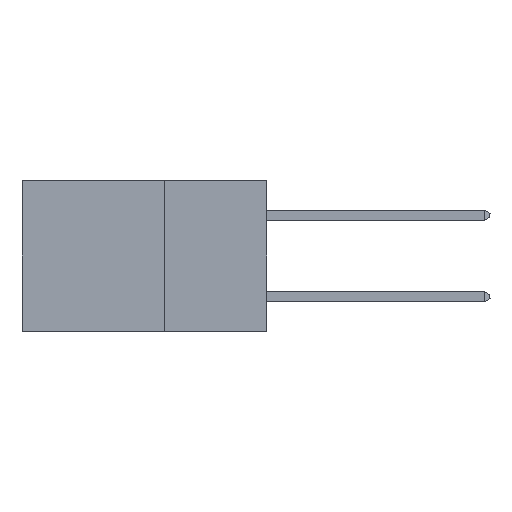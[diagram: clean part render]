
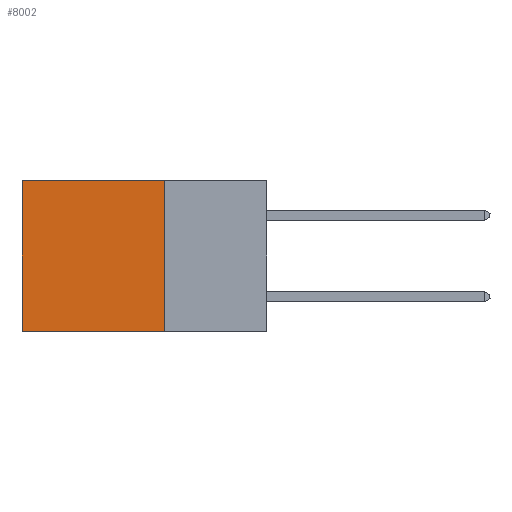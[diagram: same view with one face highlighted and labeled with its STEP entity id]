
A CAD part, left-side view. The second image highlights one B-rep face of the part: STEP entity #8002.
In plain terms, the highlighted planar face has unit normal (-1, 0, 0).
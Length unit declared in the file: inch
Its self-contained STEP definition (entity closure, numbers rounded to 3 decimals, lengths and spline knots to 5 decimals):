
#333 = DIRECTION ( 'NONE',  ( 0., 0., -1. ) ) ;
#363 = VERTEX_POINT ( 'NONE', #15415 ) ;
#1330 = ORIENTED_EDGE ( 'NONE', *, *, #5428, .T. ) ;
#1715 = DIRECTION ( 'NONE',  ( 0., 1., 0. ) ) ;
#1804 = VECTOR ( 'NONE', #1857, 39.37008 ) ;
#1857 = DIRECTION ( 'NONE',  ( 0., 0., -1. ) ) ;
#1871 = VERTEX_POINT ( 'NONE', #3184 ) ;
#2677 = LINE ( 'NONE', #12486, #1804 ) ;
#3184 = CARTESIAN_POINT ( 'NONE',  ( 0.2875, 0.25, 0. ) ) ;
#3220 = EDGE_CURVE ( 'NONE', #11445, #363, #10912, .T. ) ;
#3575 = VERTEX_POINT ( 'NONE', #6462 ) ;
#5428 = EDGE_CURVE ( 'NONE', #3575, #363, #2677, .T. ) ;
#6144 = AXIS2_PLACEMENT_3D ( 'NONE', #7206, #8565, #333 ) ;
#6462 = CARTESIAN_POINT ( 'NONE',  ( 0.2875, 0.6, 0. ) ) ;
#6562 = DIRECTION ( 'NONE',  ( 0., 1., 0. ) ) ;
#7206 = CARTESIAN_POINT ( 'NONE',  ( 0.2875, 0.25, 0. ) ) ;
#7434 = VECTOR ( 'NONE', #1715, 39.37008 ) ;
#8002 = ADVANCED_FACE ( 'NONE', ( #15183 ), #15012, .F. ) ;
#8175 = EDGE_CURVE ( 'NONE', #1871, #11445, #12346, .T. ) ;
#8340 = ORIENTED_EDGE ( 'NONE', *, *, #3220, .F. ) ;
#8398 = CARTESIAN_POINT ( 'NONE',  ( 0.2875, 0.25, -0.37 ) ) ;
#8565 = DIRECTION ( 'NONE',  ( 1., 0., 0. ) ) ;
#8910 = CARTESIAN_POINT ( 'NONE',  ( 0.2875, 0.25, 0. ) ) ;
#8911 = ORIENTED_EDGE ( 'NONE', *, *, #8175, .F. ) ;
#8918 = VECTOR ( 'NONE', #16651, 39.37008 ) ;
#10912 = LINE ( 'NONE', #13652, #7434 ) ;
#11445 = VERTEX_POINT ( 'NONE', #8398 ) ;
#12346 = LINE ( 'NONE', #8910, #8918 ) ;
#12450 = EDGE_CURVE ( 'NONE', #1871, #3575, #17234, .T. ) ;
#12486 = CARTESIAN_POINT ( 'NONE',  ( 0.2875, 0.6, 0. ) ) ;
#13074 = CARTESIAN_POINT ( 'NONE',  ( 0.2875, 0.25, 0. ) ) ;
#13652 = CARTESIAN_POINT ( 'NONE',  ( 0.2875, 0.25, -0.37 ) ) ;
#13815 = VECTOR ( 'NONE', #6562, 39.37008 ) ;
#14297 = ORIENTED_EDGE ( 'NONE', *, *, #12450, .T. ) ;
#15012 = PLANE ( 'NONE',  #6144 ) ;
#15183 = FACE_OUTER_BOUND ( 'NONE', #15537, .T. ) ;
#15415 = CARTESIAN_POINT ( 'NONE',  ( 0.2875, 0.6, -0.37 ) ) ;
#15537 = EDGE_LOOP ( 'NONE', ( #1330, #8340, #8911, #14297 ) ) ;
#16651 = DIRECTION ( 'NONE',  ( 0., 0., -1. ) ) ;
#17234 = LINE ( 'NONE', #13074, #13815 ) ;
